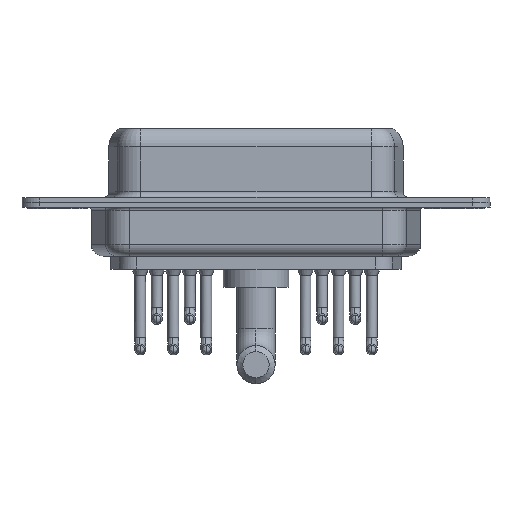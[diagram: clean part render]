
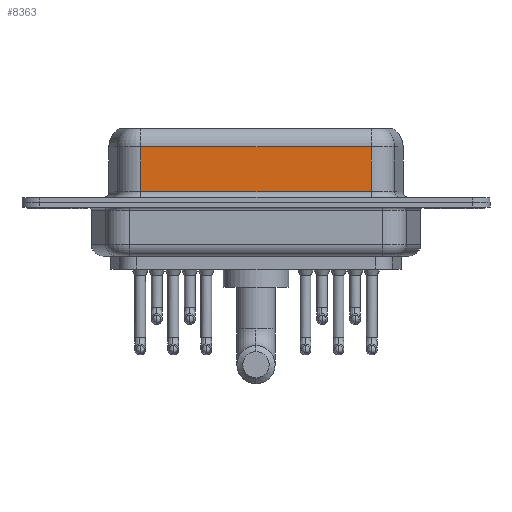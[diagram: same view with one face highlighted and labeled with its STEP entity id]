
A CAD part, front view. The second image highlights one B-rep face of the part: STEP entity #8363.
In plain terms, the highlighted planar face has unit normal (0, -1, 0).
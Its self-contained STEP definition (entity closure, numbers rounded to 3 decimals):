
#39 = ORIENTED_EDGE ( 'NONE', *, *, #3563, .T. ) ;
#545 = ORIENTED_EDGE ( 'NONE', *, *, #12299, .T. ) ;
#2130 = VERTEX_POINT ( 'NONE', #5624 ) ;
#2377 = LINE ( 'NONE', #15284, #5275 ) ;
#3026 = DIRECTION ( 'NONE',  ( 0., 1., 0. ) ) ;
#3177 = LINE ( 'NONE', #10789, #6225 ) ;
#3563 = EDGE_CURVE ( 'NONE', #2130, #13251, #13810, .T. ) ;
#3733 = DIRECTION ( 'NONE',  ( 0., 0., -1. ) ) ;
#4341 = EDGE_CURVE ( 'NONE', #15291, #11056, #2377, .T. ) ;
#4384 = DIRECTION ( 'NONE',  ( 0., 0., -1. ) ) ;
#4404 = FACE_OUTER_BOUND ( 'NONE', #4455, .T. ) ;
#4455 = EDGE_LOOP ( 'NONE', ( #5833, #39, #545, #12345 ) ) ;
#5275 = VECTOR ( 'NONE', #9818, 1000. ) ;
#5624 = CARTESIAN_POINT ( 'NONE',  ( 26.287, -3.95, 4.65 ) ) ;
#5662 = CARTESIAN_POINT ( 'NONE',  ( 26.287, -3.95, 0.9 ) ) ;
#5833 = ORIENTED_EDGE ( 'NONE', *, *, #15468, .F. ) ;
#6225 = VECTOR ( 'NONE', #4384, 1000. ) ;
#7150 = CARTESIAN_POINT ( 'NONE',  ( 7.013, -3.95, 4.65 ) ) ;
#8363 = ADVANCED_FACE ( 'NONE', ( #4404 ), #13622, .F. ) ;
#8437 = CARTESIAN_POINT ( 'NONE',  ( 26.287, -3.95, 4.65 ) ) ;
#8610 = DIRECTION ( 'NONE',  ( -1., 0., 0. ) ) ;
#9597 = CARTESIAN_POINT ( 'NONE',  ( 26.287, -3.95, 6.4 ) ) ;
#9818 = DIRECTION ( 'NONE',  ( 1., 0., 0. ) ) ;
#10789 = CARTESIAN_POINT ( 'NONE',  ( 7.013, -3.95, 6.4 ) ) ;
#11056 = VERTEX_POINT ( 'NONE', #5662 ) ;
#12299 = EDGE_CURVE ( 'NONE', #13251, #15291, #3177, .T. ) ;
#12335 = DIRECTION ( 'NONE',  ( 0., 0., 1. ) ) ;
#12345 = ORIENTED_EDGE ( 'NONE', *, *, #4341, .T. ) ;
#13251 = VERTEX_POINT ( 'NONE', #7150 ) ;
#13486 = VECTOR ( 'NONE', #8610, 1000. ) ;
#13500 = AXIS2_PLACEMENT_3D ( 'NONE', #9597, #3026, #12335 ) ;
#13622 = PLANE ( 'NONE',  #13500 ) ;
#13810 = LINE ( 'NONE', #8437, #13486 ) ;
#15284 = CARTESIAN_POINT ( 'NONE',  ( 26.287, -3.95, 0.9 ) ) ;
#15291 = VERTEX_POINT ( 'NONE', #16551 ) ;
#15468 = EDGE_CURVE ( 'NONE', #2130, #11056, #15510, .T. ) ;
#15510 = LINE ( 'NONE', #16633, #16677 ) ;
#16551 = CARTESIAN_POINT ( 'NONE',  ( 7.013, -3.95, 0.9 ) ) ;
#16633 = CARTESIAN_POINT ( 'NONE',  ( 26.287, -3.95, 6.4 ) ) ;
#16677 = VECTOR ( 'NONE', #3733, 1000. ) ;
